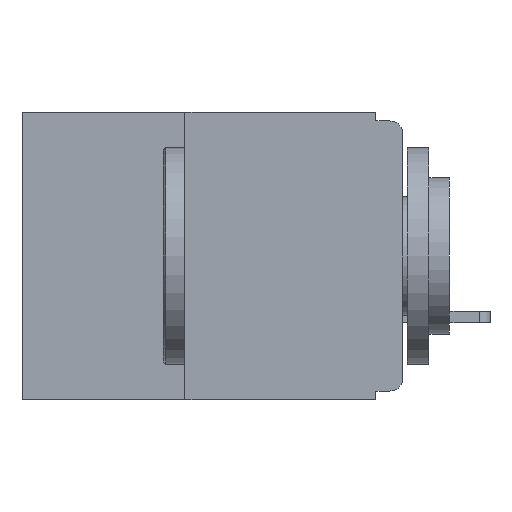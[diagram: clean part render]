
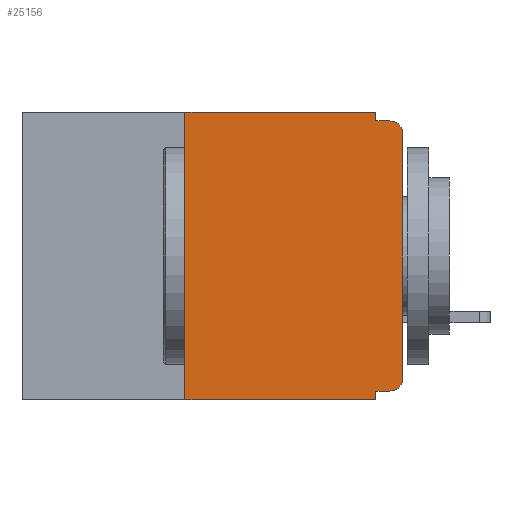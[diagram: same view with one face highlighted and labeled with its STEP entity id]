
A CAD part, left-side view. The second image highlights one B-rep face of the part: STEP entity #25156.
In plain terms, the highlighted planar face has unit normal (-1, 0, 0).
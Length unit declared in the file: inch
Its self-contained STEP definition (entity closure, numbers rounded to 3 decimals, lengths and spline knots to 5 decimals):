
#1662 = CARTESIAN_POINT ( 'NONE',  ( 0., 0.25, 0. ) ) ;
#1859 = PLANE ( 'NONE',  #17279 ) ;
#1989 = VECTOR ( 'NONE', #5353, 39.37008 ) ;
#2023 = EDGE_CURVE ( 'NONE', #27750, #27122, #3077, .T. ) ;
#2628 = DIRECTION ( 'NONE',  ( -1., 0., 0. ) ) ;
#2845 = DIRECTION ( 'NONE',  ( -1., 0., 0. ) ) ;
#3077 = LINE ( 'NONE', #15094, #22158 ) ;
#4106 = CARTESIAN_POINT ( 'NONE',  ( 0., 0.437, 0. ) ) ;
#4304 = DIRECTION ( 'NONE',  ( 1., 0., 0. ) ) ;
#4833 = CARTESIAN_POINT ( 'NONE',  ( 0., 0., -0.01 ) ) ;
#5353 = DIRECTION ( 'NONE',  ( 0., -1., 0. ) ) ;
#5686 = ORIENTED_EDGE ( 'NONE', *, *, #29157, .T. ) ;
#5848 = LINE ( 'NONE', #11648, #24056 ) ;
#6216 = VECTOR ( 'NONE', #18942, 39.37008 ) ;
#6813 = VERTEX_POINT ( 'NONE', #11079 ) ;
#7016 = CARTESIAN_POINT ( 'NONE',  ( 0., 0., -0.305 ) ) ;
#7130 = CIRCLE ( 'NONE', #27969, 0.015 ) ;
#7197 = EDGE_LOOP ( 'NONE', ( #5686, #29581, #11067, #24832, #27932, #10487, #21868, #13078, #22109, #25638 ) ) ;
#7230 = CARTESIAN_POINT ( 'NONE',  ( 0., 0., -0.32 ) ) ;
#8846 = EDGE_CURVE ( 'NONE', #27939, #30104, #11862, .T. ) ;
#9200 = EDGE_CURVE ( 'NONE', #10091, #27750, #21103, .T. ) ;
#9349 = DIRECTION ( 'NONE',  ( 0., 0., -1. ) ) ;
#9576 = CARTESIAN_POINT ( 'NONE',  ( 0., 0.015, -0.01 ) ) ;
#10014 = LINE ( 'NONE', #21173, #24080 ) ;
#10091 = VERTEX_POINT ( 'NONE', #1662 ) ;
#10136 = DIRECTION ( 'NONE',  ( 0., 0., 1. ) ) ;
#10487 = ORIENTED_EDGE ( 'NONE', *, *, #23089, .F. ) ;
#11023 = LINE ( 'NONE', #7230, #22889 ) ;
#11067 = ORIENTED_EDGE ( 'NONE', *, *, #12082, .F. ) ;
#11079 = CARTESIAN_POINT ( 'NONE',  ( 0., 0.031, -0.32 ) ) ;
#11467 = AXIS2_PLACEMENT_3D ( 'NONE', #17048, #2628, #19420 ) ;
#11648 = CARTESIAN_POINT ( 'NONE',  ( 0., 0., 0. ) ) ;
#11691 = VERTEX_POINT ( 'NONE', #12979 ) ;
#11862 = LINE ( 'NONE', #17536, #6216 ) ;
#12013 = CARTESIAN_POINT ( 'NONE',  ( 0., 0.031, 0. ) ) ;
#12082 = EDGE_CURVE ( 'NONE', #27122, #12402, #15573, .T. ) ;
#12402 = VERTEX_POINT ( 'NONE', #9576 ) ;
#12979 = CARTESIAN_POINT ( 'NONE',  ( 0., 0., -0.025 ) ) ;
#13032 = EDGE_CURVE ( 'NONE', #20622, #6813, #11023, .T. ) ;
#13078 = ORIENTED_EDGE ( 'NONE', *, *, #28844, .F. ) ;
#14058 = DIRECTION ( 'NONE',  ( 0., 0., 1. ) ) ;
#14921 = EDGE_CURVE ( 'NONE', #11691, #12402, #7130, .T. ) ;
#15094 = CARTESIAN_POINT ( 'NONE',  ( 0., 0.031, 0. ) ) ;
#15320 = DIRECTION ( 'NONE',  ( 0., 0., -1. ) ) ;
#15573 = LINE ( 'NONE', #4833, #27996 ) ;
#15776 = EDGE_CURVE ( 'NONE', #20622, #27088, #27063, .T. ) ;
#17048 = CARTESIAN_POINT ( 'NONE',  ( 0., 0.015, -0.305 ) ) ;
#17269 = CARTESIAN_POINT ( 'NONE',  ( 0., 0.015, -0.025 ) ) ;
#17279 = AXIS2_PLACEMENT_3D ( 'NONE', #25623, #4304, #21037 ) ;
#17536 = CARTESIAN_POINT ( 'NONE',  ( 0., 0.437, -0.33 ) ) ;
#18942 = DIRECTION ( 'NONE',  ( 0., -1., 0. ) ) ;
#19134 = DIRECTION ( 'NONE',  ( 0., 1., 0. ) ) ;
#19420 = DIRECTION ( 'NONE',  ( 0., 0., -1. ) ) ;
#19487 = VECTOR ( 'NONE', #10136, 39.37008 ) ;
#19645 = DIRECTION ( 'NONE',  ( 0., 0., -1. ) ) ;
#20229 = LINE ( 'NONE', #21947, #19487 ) ;
#20622 = VERTEX_POINT ( 'NONE', #25208 ) ;
#21037 = DIRECTION ( 'NONE',  ( 0., 0., -1. ) ) ;
#21103 = LINE ( 'NONE', #4106, #1989 ) ;
#21173 = CARTESIAN_POINT ( 'NONE',  ( 0., 0.031, -0.33 ) ) ;
#21527 = DIRECTION ( 'NONE',  ( 0., -1., 0. ) ) ;
#21868 = ORIENTED_EDGE ( 'NONE', *, *, #8846, .T. ) ;
#21947 = CARTESIAN_POINT ( 'NONE',  ( 0., 0.25, -0.33 ) ) ;
#22109 = ORIENTED_EDGE ( 'NONE', *, *, #13032, .F. ) ;
#22158 = VECTOR ( 'NONE', #15320, 39.37008 ) ;
#22889 = VECTOR ( 'NONE', #19134, 39.37008 ) ;
#23089 = EDGE_CURVE ( 'NONE', #27939, #10091, #20229, .T. ) ;
#24056 = VECTOR ( 'NONE', #14058, 39.37008 ) ;
#24080 = VECTOR ( 'NONE', #9349, 39.37008 ) ;
#24800 = CARTESIAN_POINT ( 'NONE',  ( 0., 0.031, -0.33 ) ) ;
#24832 = ORIENTED_EDGE ( 'NONE', *, *, #2023, .F. ) ;
#25156 = ADVANCED_FACE ( 'NONE', ( #30383 ), #1859, .F. ) ;
#25208 = CARTESIAN_POINT ( 'NONE',  ( 0., 0.015, -0.32 ) ) ;
#25623 = CARTESIAN_POINT ( 'NONE',  ( 0., 0.437, 0. ) ) ;
#25638 = ORIENTED_EDGE ( 'NONE', *, *, #15776, .T. ) ;
#27063 = CIRCLE ( 'NONE', #11467, 0.015 ) ;
#27088 = VERTEX_POINT ( 'NONE', #7016 ) ;
#27122 = VERTEX_POINT ( 'NONE', #28349 ) ;
#27750 = VERTEX_POINT ( 'NONE', #12013 ) ;
#27932 = ORIENTED_EDGE ( 'NONE', *, *, #9200, .F. ) ;
#27939 = VERTEX_POINT ( 'NONE', #29102 ) ;
#27969 = AXIS2_PLACEMENT_3D ( 'NONE', #17269, #2845, #19645 ) ;
#27996 = VECTOR ( 'NONE', #21527, 39.37008 ) ;
#28349 = CARTESIAN_POINT ( 'NONE',  ( 0., 0.031, -0.01 ) ) ;
#28844 = EDGE_CURVE ( 'NONE', #6813, #30104, #10014, .T. ) ;
#29102 = CARTESIAN_POINT ( 'NONE',  ( 0., 0.25, -0.33 ) ) ;
#29157 = EDGE_CURVE ( 'NONE', #27088, #11691, #5848, .T. ) ;
#29581 = ORIENTED_EDGE ( 'NONE', *, *, #14921, .T. ) ;
#30104 = VERTEX_POINT ( 'NONE', #24800 ) ;
#30383 = FACE_OUTER_BOUND ( 'NONE', #7197, .T. ) ;
